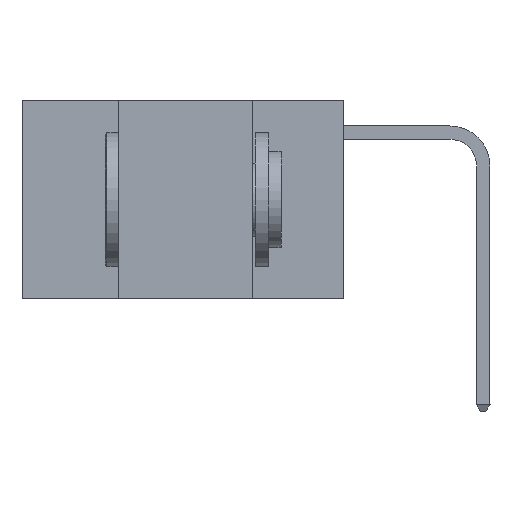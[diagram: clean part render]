
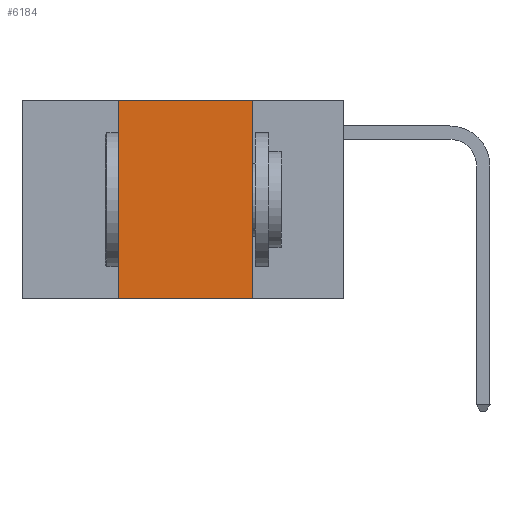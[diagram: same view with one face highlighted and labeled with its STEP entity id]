
A CAD part, left-side view. The second image highlights one B-rep face of the part: STEP entity #6184.
In plain terms, the highlighted planar face has unit normal (-1, 0, 0).
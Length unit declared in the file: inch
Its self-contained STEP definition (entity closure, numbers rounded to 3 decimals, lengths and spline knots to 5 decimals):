
#1125 = LINE ( 'NONE', #5959, #11982 ) ;
#1189 = DIRECTION ( 'NONE',  ( 1., 0., 0. ) ) ;
#1668 = VERTEX_POINT ( 'NONE', #11692 ) ;
#2135 = CARTESIAN_POINT ( 'NONE',  ( 0., 0.17, 0. ) ) ;
#2440 = CARTESIAN_POINT ( 'NONE',  ( 0., 0.17, -0.37 ) ) ;
#3696 = VERTEX_POINT ( 'NONE', #13591 ) ;
#4282 = ORIENTED_EDGE ( 'NONE', *, *, #13753, .F. ) ;
#4376 = VERTEX_POINT ( 'NONE', #2440 ) ;
#4495 = ORIENTED_EDGE ( 'NONE', *, *, #4730, .F. ) ;
#4622 = LINE ( 'NONE', #7927, #7945 ) ;
#4730 = EDGE_CURVE ( 'NONE', #1668, #3696, #1125, .T. ) ;
#5029 = VERTEX_POINT ( 'NONE', #12493 ) ;
#5637 = EDGE_LOOP ( 'NONE', ( #10150, #4495, #4282, #12892 ) ) ;
#5959 = CARTESIAN_POINT ( 'NONE',  ( 0., 0.6, 0. ) ) ;
#6184 = ADVANCED_FACE ( 'NONE', ( #13998 ), #8131, .F. ) ;
#7927 = CARTESIAN_POINT ( 'NONE',  ( 0., 0.6, -0.37 ) ) ;
#7945 = VECTOR ( 'NONE', #13716, 39.37008 ) ;
#7990 = DIRECTION ( 'NONE',  ( 0., 0., 1. ) ) ;
#8131 = PLANE ( 'NONE',  #12717 ) ;
#8442 = DIRECTION ( 'NONE',  ( 0., 0., -1. ) ) ;
#8818 = VECTOR ( 'NONE', #7990, 39.37008 ) ;
#10135 = LINE ( 'NONE', #11300, #8818 ) ;
#10150 = ORIENTED_EDGE ( 'NONE', *, *, #13789, .F. ) ;
#10376 = DIRECTION ( 'NONE',  ( 0., 0., -1. ) ) ;
#11300 = CARTESIAN_POINT ( 'NONE',  ( 0., 0.42, 0. ) ) ;
#11534 = DIRECTION ( 'NONE',  ( 0., -1., 0. ) ) ;
#11692 = CARTESIAN_POINT ( 'NONE',  ( 0., 0.42, 0. ) ) ;
#11982 = VECTOR ( 'NONE', #11534, 39.37008 ) ;
#12493 = CARTESIAN_POINT ( 'NONE',  ( 0., 0.42, -0.37 ) ) ;
#12677 = LINE ( 'NONE', #2135, #14002 ) ;
#12717 = AXIS2_PLACEMENT_3D ( 'NONE', #14293, #1189, #8442 ) ;
#12892 = ORIENTED_EDGE ( 'NONE', *, *, #13405, .T. ) ;
#13405 = EDGE_CURVE ( 'NONE', #5029, #4376, #4622, .T. ) ;
#13591 = CARTESIAN_POINT ( 'NONE',  ( 0., 0.17, 0. ) ) ;
#13716 = DIRECTION ( 'NONE',  ( 0., -1., 0. ) ) ;
#13753 = EDGE_CURVE ( 'NONE', #5029, #1668, #10135, .T. ) ;
#13789 = EDGE_CURVE ( 'NONE', #3696, #4376, #12677, .T. ) ;
#13998 = FACE_OUTER_BOUND ( 'NONE', #5637, .T. ) ;
#14002 = VECTOR ( 'NONE', #10376, 39.37008 ) ;
#14293 = CARTESIAN_POINT ( 'NONE',  ( 0., 0.6, 0. ) ) ;
